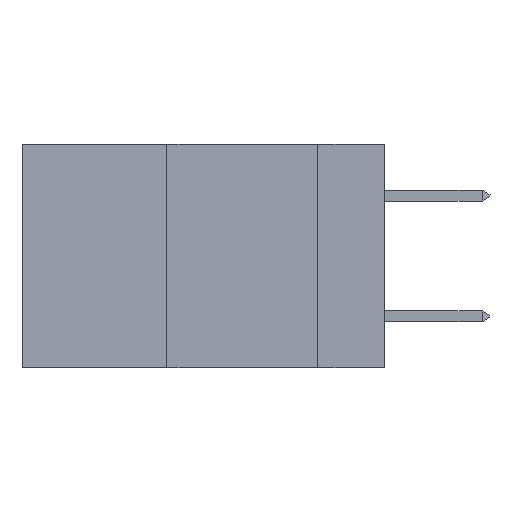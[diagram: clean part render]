
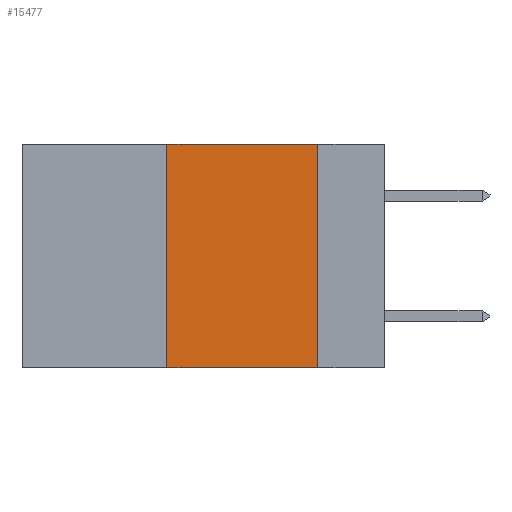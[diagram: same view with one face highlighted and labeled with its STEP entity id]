
A CAD part, left-side view. The second image highlights one B-rep face of the part: STEP entity #15477.
In plain terms, the highlighted planar face has unit normal (-1, 0, 0).
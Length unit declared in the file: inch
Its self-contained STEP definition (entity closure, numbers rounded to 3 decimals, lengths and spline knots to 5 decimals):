
#301 = LINE ( 'NONE', #2440, #10497 ) ;
#1315 = VERTEX_POINT ( 'NONE', #21123 ) ;
#1472 = CARTESIAN_POINT ( 'NONE',  ( 0., 0.6, 0. ) ) ;
#2078 = CARTESIAN_POINT ( 'NONE',  ( 0., 0.11, 0. ) ) ;
#2201 = VECTOR ( 'NONE', #6659, 39.37008 ) ;
#2440 = CARTESIAN_POINT ( 'NONE',  ( 0., 0.6, 0. ) ) ;
#2450 = AXIS2_PLACEMENT_3D ( 'NONE', #1472, #19927, #16648 ) ;
#2658 = VERTEX_POINT ( 'NONE', #6733 ) ;
#3754 = DIRECTION ( 'NONE',  ( 0., 0., -1. ) ) ;
#5935 = ORIENTED_EDGE ( 'NONE', *, *, #18371, .F. ) ;
#6067 = DIRECTION ( 'NONE',  ( 0., -1., 0. ) ) ;
#6659 = DIRECTION ( 'NONE',  ( 0., 0., 1. ) ) ;
#6733 = CARTESIAN_POINT ( 'NONE',  ( 0., 0.36, -0.37 ) ) ;
#6864 = ORIENTED_EDGE ( 'NONE', *, *, #9390, .T. ) ;
#7483 = LINE ( 'NONE', #2078, #18127 ) ;
#8390 = CARTESIAN_POINT ( 'NONE',  ( 0., 0.11, -0.37 ) ) ;
#8429 = ORIENTED_EDGE ( 'NONE', *, *, #10425, .F. ) ;
#8842 = ORIENTED_EDGE ( 'NONE', *, *, #16842, .F. ) ;
#9390 = EDGE_CURVE ( 'NONE', #2658, #19710, #17535, .T. ) ;
#10163 = VERTEX_POINT ( 'NONE', #11688 ) ;
#10425 = EDGE_CURVE ( 'NONE', #10163, #19710, #7483, .T. ) ;
#10497 = VECTOR ( 'NONE', #6067, 39.37008 ) ;
#11688 = CARTESIAN_POINT ( 'NONE',  ( 0., 0.11, 0. ) ) ;
#12005 = DIRECTION ( 'NONE',  ( 0., -1., 0. ) ) ;
#12952 = EDGE_LOOP ( 'NONE', ( #8429, #5935, #8842, #6864 ) ) ;
#14514 = LINE ( 'NONE', #19959, #2201 ) ;
#14723 = PLANE ( 'NONE',  #2450 ) ;
#15477 = ADVANCED_FACE ( 'NONE', ( #19183 ), #14723, .F. ) ;
#16248 = VECTOR ( 'NONE', #12005, 39.37008 ) ;
#16648 = DIRECTION ( 'NONE',  ( 0., 0., -1. ) ) ;
#16842 = EDGE_CURVE ( 'NONE', #2658, #1315, #14514, .T. ) ;
#16905 = CARTESIAN_POINT ( 'NONE',  ( 0., 0.6, -0.37 ) ) ;
#17535 = LINE ( 'NONE', #16905, #16248 ) ;
#18127 = VECTOR ( 'NONE', #3754, 39.37008 ) ;
#18371 = EDGE_CURVE ( 'NONE', #1315, #10163, #301, .T. ) ;
#19183 = FACE_OUTER_BOUND ( 'NONE', #12952, .T. ) ;
#19710 = VERTEX_POINT ( 'NONE', #8390 ) ;
#19927 = DIRECTION ( 'NONE',  ( 1., 0., 0. ) ) ;
#19959 = CARTESIAN_POINT ( 'NONE',  ( 0., 0.36, 0. ) ) ;
#21123 = CARTESIAN_POINT ( 'NONE',  ( 0., 0.36, 0. ) ) ;
